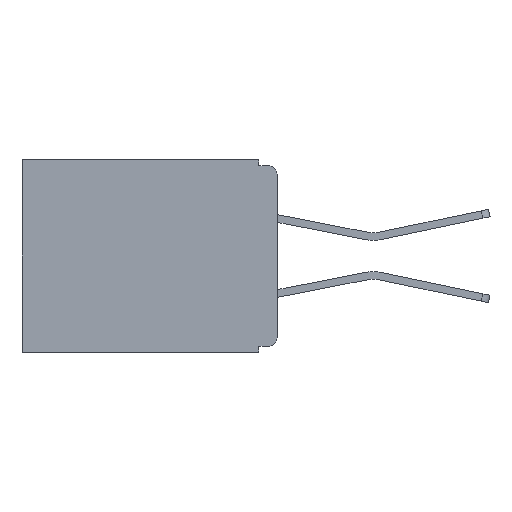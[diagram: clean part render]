
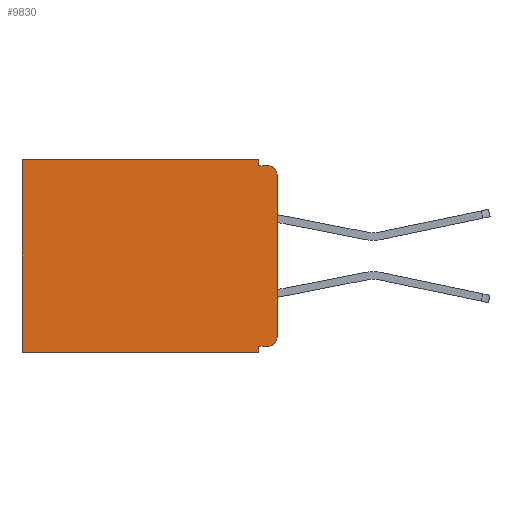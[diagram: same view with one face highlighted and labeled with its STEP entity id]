
A CAD part, left-side view. The second image highlights one B-rep face of the part: STEP entity #9830.
In plain terms, the highlighted planar face has unit normal (-1, 0, 0).
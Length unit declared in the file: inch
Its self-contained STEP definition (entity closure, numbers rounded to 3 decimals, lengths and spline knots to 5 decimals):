
#28 = ORIENTED_EDGE ( 'NONE', *, *, #10769, .T. ) ;
#71 = EDGE_CURVE ( 'NONE', #14369, #21465, #6599, .T. ) ;
#166 = CARTESIAN_POINT ( 'NONE',  ( 0.3, 0.015, -0.32 ) ) ;
#635 = ORIENTED_EDGE ( 'NONE', *, *, #18796, .F. ) ;
#995 = EDGE_CURVE ( 'NONE', #16645, #21072, #21235, .T. ) ;
#1412 = VECTOR ( 'NONE', #2206, 39.37008 ) ;
#1911 = CARTESIAN_POINT ( 'NONE',  ( 0.3, 0.437, 0. ) ) ;
#2188 = DIRECTION ( 'NONE',  ( 0., 1., 0. ) ) ;
#2206 = DIRECTION ( 'NONE',  ( 0., 1., 0. ) ) ;
#2402 = DIRECTION ( 'NONE',  ( 0., -1., 0. ) ) ;
#2649 = LINE ( 'NONE', #24219, #5939 ) ;
#2783 = ORIENTED_EDGE ( 'NONE', *, *, #5676, .T. ) ;
#2860 = VECTOR ( 'NONE', #17795, 39.37008 ) ;
#3462 = LINE ( 'NONE', #15856, #2860 ) ;
#3903 = VERTEX_POINT ( 'NONE', #166 ) ;
#4288 = ORIENTED_EDGE ( 'NONE', *, *, #71, .T. ) ;
#4334 = CARTESIAN_POINT ( 'NONE',  ( 0.3, 0., -0.01 ) ) ;
#4869 = CARTESIAN_POINT ( 'NONE',  ( 0.3, 0., -0.305 ) ) ;
#5257 = CARTESIAN_POINT ( 'NONE',  ( 0.3, 0., -0.33 ) ) ;
#5312 = CARTESIAN_POINT ( 'NONE',  ( 0.3, 0.031, -0.01 ) ) ;
#5421 = LINE ( 'NONE', #24746, #19608 ) ;
#5542 = AXIS2_PLACEMENT_3D ( 'NONE', #9322, #20329, #20097 ) ;
#5676 = EDGE_CURVE ( 'NONE', #12681, #6688, #8508, .T. ) ;
#5835 = DIRECTION ( 'NONE',  ( 0., 0., -1. ) ) ;
#5862 = DIRECTION ( 'NONE',  ( -1., 0., 0. ) ) ;
#5868 = CARTESIAN_POINT ( 'NONE',  ( 0.3, 0.015, -0.305 ) ) ;
#5921 = VECTOR ( 'NONE', #2188, 39.37008 ) ;
#5939 = VECTOR ( 'NONE', #16720, 39.37008 ) ;
#5958 = DIRECTION ( 'NONE',  ( 0., 0., -1. ) ) ;
#6334 = EDGE_CURVE ( 'NONE', #14369, #17203, #5421, .T. ) ;
#6596 = CARTESIAN_POINT ( 'NONE',  ( 0.3, 0.437, -0.33 ) ) ;
#6599 = LINE ( 'NONE', #16112, #1412 ) ;
#6688 = VERTEX_POINT ( 'NONE', #24752 ) ;
#6732 = ORIENTED_EDGE ( 'NONE', *, *, #995, .F. ) ;
#6845 = LINE ( 'NONE', #24809, #21547 ) ;
#7315 = ORIENTED_EDGE ( 'NONE', *, *, #18153, .F. ) ;
#7353 = DIRECTION ( 'NONE',  ( 0., 0., -1. ) ) ;
#7612 = ORIENTED_EDGE ( 'NONE', *, *, #6334, .F. ) ;
#8508 = CIRCLE ( 'NONE', #5542, 0.015 ) ;
#8853 = LINE ( 'NONE', #4334, #22901 ) ;
#9011 = CARTESIAN_POINT ( 'NONE',  ( 0.3, 0.031, -0.33 ) ) ;
#9322 = CARTESIAN_POINT ( 'NONE',  ( 0.3, 0.015, -0.025 ) ) ;
#9542 = DIRECTION ( 'NONE',  ( 0., 0., -1. ) ) ;
#9741 = ORIENTED_EDGE ( 'NONE', *, *, #12475, .F. ) ;
#9830 = ADVANCED_FACE ( 'NONE', ( #12414 ), #17134, .F. ) ;
#9854 = CARTESIAN_POINT ( 'NONE',  ( 0.3, 0.437, -0.33 ) ) ;
#10044 = ORIENTED_EDGE ( 'NONE', *, *, #13384, .T. ) ;
#10769 = EDGE_CURVE ( 'NONE', #3903, #12992, #15101, .T. ) ;
#11027 = LINE ( 'NONE', #9854, #15556 ) ;
#12414 = FACE_OUTER_BOUND ( 'NONE', #18867, .T. ) ;
#12475 = EDGE_CURVE ( 'NONE', #3903, #23067, #2649, .T. ) ;
#12681 = VERTEX_POINT ( 'NONE', #22981 ) ;
#12992 = VERTEX_POINT ( 'NONE', #4869 ) ;
#13384 = EDGE_CURVE ( 'NONE', #21465, #21072, #11027, .T. ) ;
#14369 = VERTEX_POINT ( 'NONE', #22726 ) ;
#14538 = ORIENTED_EDGE ( 'NONE', *, *, #16210, .F. ) ;
#15101 = CIRCLE ( 'NONE', #20961, 0.015 ) ;
#15556 = VECTOR ( 'NONE', #5958, 39.37008 ) ;
#15856 = CARTESIAN_POINT ( 'NONE',  ( 0.3, 0.031, -0.33 ) ) ;
#16112 = CARTESIAN_POINT ( 'NONE',  ( 0.3, 0., 0. ) ) ;
#16210 = EDGE_CURVE ( 'NONE', #12681, #12992, #6845, .T. ) ;
#16645 = VERTEX_POINT ( 'NONE', #9011 ) ;
#16720 = DIRECTION ( 'NONE',  ( 0., 1., 0. ) ) ;
#17053 = DIRECTION ( 'NONE',  ( 0., 0., -1. ) ) ;
#17073 = DIRECTION ( 'NONE',  ( 1., 0., 0. ) ) ;
#17134 = PLANE ( 'NONE',  #19866 ) ;
#17182 = CARTESIAN_POINT ( 'NONE',  ( 0.3, 0., -0.33 ) ) ;
#17203 = VERTEX_POINT ( 'NONE', #5312 ) ;
#17795 = DIRECTION ( 'NONE',  ( 0., 0., -1. ) ) ;
#18153 = EDGE_CURVE ( 'NONE', #23067, #16645, #3462, .T. ) ;
#18796 = EDGE_CURVE ( 'NONE', #17203, #6688, #8853, .T. ) ;
#18867 = EDGE_LOOP ( 'NONE', ( #14538, #2783, #635, #7612, #4288, #10044, #6732, #7315, #9741, #28 ) ) ;
#19608 = VECTOR ( 'NONE', #7353, 39.37008 ) ;
#19866 = AXIS2_PLACEMENT_3D ( 'NONE', #17182, #17073, #17053 ) ;
#20097 = DIRECTION ( 'NONE',  ( 0., 0., -1. ) ) ;
#20329 = DIRECTION ( 'NONE',  ( -1., 0., 0. ) ) ;
#20961 = AXIS2_PLACEMENT_3D ( 'NONE', #5868, #5862, #5835 ) ;
#21072 = VERTEX_POINT ( 'NONE', #6596 ) ;
#21235 = LINE ( 'NONE', #5257, #5921 ) ;
#21465 = VERTEX_POINT ( 'NONE', #1911 ) ;
#21547 = VECTOR ( 'NONE', #9542, 39.37008 ) ;
#22726 = CARTESIAN_POINT ( 'NONE',  ( 0.3, 0.031, 0. ) ) ;
#22901 = VECTOR ( 'NONE', #2402, 39.37008 ) ;
#22981 = CARTESIAN_POINT ( 'NONE',  ( 0.3, 0., -0.025 ) ) ;
#23067 = VERTEX_POINT ( 'NONE', #24272 ) ;
#24219 = CARTESIAN_POINT ( 'NONE',  ( 0.3, 0., -0.32 ) ) ;
#24272 = CARTESIAN_POINT ( 'NONE',  ( 0.3, 0.031, -0.32 ) ) ;
#24746 = CARTESIAN_POINT ( 'NONE',  ( 0.3, 0.031, 0. ) ) ;
#24752 = CARTESIAN_POINT ( 'NONE',  ( 0.3, 0.015, -0.01 ) ) ;
#24809 = CARTESIAN_POINT ( 'NONE',  ( 0.3, 0., -0.33 ) ) ;
